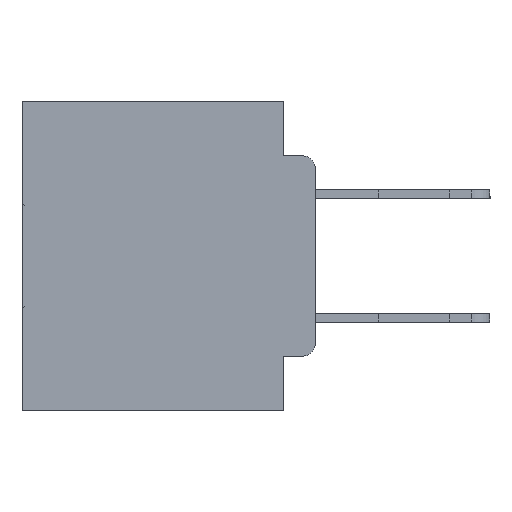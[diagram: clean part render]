
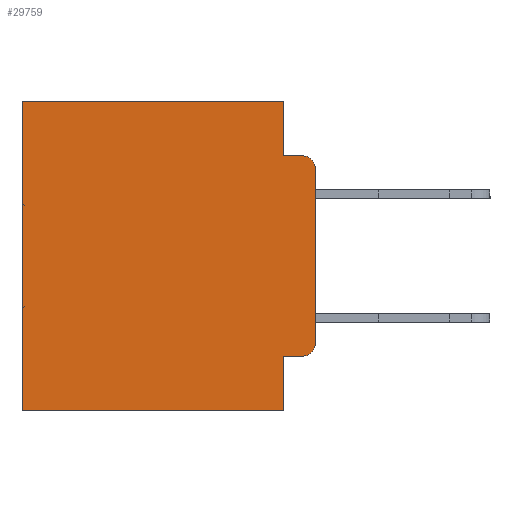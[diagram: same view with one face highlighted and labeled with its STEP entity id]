
A CAD part, left-side view. The second image highlights one B-rep face of the part: STEP entity #29759.
In plain terms, the highlighted planar face has unit normal (-1, 0, 0).
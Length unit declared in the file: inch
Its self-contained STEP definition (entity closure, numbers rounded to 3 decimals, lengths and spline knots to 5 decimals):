
#128 = EDGE_CURVE ( 'NONE', #27469, #11849, #14133, .T. ) ;
#527 = EDGE_CURVE ( 'NONE', #28524, #11849, #22527, .T. ) ;
#592 = VECTOR ( 'NONE', #29927, 39.37008 ) ;
#856 = PLANE ( 'NONE',  #10819 ) ;
#978 = LINE ( 'NONE', #7928, #26305 ) ;
#1054 = EDGE_CURVE ( 'NONE', #17844, #15784, #29932, .T. ) ;
#1127 = DIRECTION ( 'NONE',  ( 0., 0., -1. ) ) ;
#1215 = VERTEX_POINT ( 'NONE', #1244 ) ;
#1244 = CARTESIAN_POINT ( 'NONE',  ( 0.298, 0.473, -0.5 ) ) ;
#1388 = EDGE_CURVE ( 'NONE', #15784, #13657, #13635, .T. ) ;
#1436 = DIRECTION ( 'NONE',  ( 0., 0., -1. ) ) ;
#1456 = LINE ( 'NONE', #21201, #28298 ) ;
#1610 = AXIS2_PLACEMENT_3D ( 'NONE', #18810, #2027, #1436 ) ;
#1756 = CARTESIAN_POINT ( 'NONE',  ( 0.298, 0., 0. ) ) ;
#2012 = EDGE_CURVE ( 'NONE', #23651, #12272, #1456, .T. ) ;
#2027 = DIRECTION ( 'NONE',  ( -1., 0., 0. ) ) ;
#3359 = CARTESIAN_POINT ( 'NONE',  ( 0.298, 0., -0.3915 ) ) ;
#5208 = CARTESIAN_POINT ( 'NONE',  ( 0.298, 0., -0.5 ) ) ;
#5231 = DIRECTION ( 'NONE',  ( 0., 1., 0. ) ) ;
#6054 = AXIS2_PLACEMENT_3D ( 'NONE', #12619, #30339, #15205 ) ;
#7904 = DIRECTION ( 'NONE',  ( 0., 1., 0. ) ) ;
#7928 = CARTESIAN_POINT ( 'NONE',  ( 0.298, 0., 0. ) ) ;
#8842 = VERTEX_POINT ( 'NONE', #31891 ) ;
#9017 = ORIENTED_EDGE ( 'NONE', *, *, #1388, .F. ) ;
#9561 = VECTOR ( 'NONE', #24460, 39.37008 ) ;
#10523 = CARTESIAN_POINT ( 'NONE',  ( 0.298, 0.02, -0.0885 ) ) ;
#10819 = AXIS2_PLACEMENT_3D ( 'NONE', #16819, #27008, #11722 ) ;
#11003 = EDGE_CURVE ( 'NONE', #23651, #27469, #25296, .T. ) ;
#11676 = VECTOR ( 'NONE', #23609, 39.37008 ) ;
#11722 = DIRECTION ( 'NONE',  ( 0., 0., -1. ) ) ;
#11849 = VERTEX_POINT ( 'NONE', #3359 ) ;
#12272 = VERTEX_POINT ( 'NONE', #17216 ) ;
#12349 = CARTESIAN_POINT ( 'NONE',  ( 0.298, 0.051, 0. ) ) ;
#12554 = EDGE_CURVE ( 'NONE', #12272, #1215, #20875, .T. ) ;
#12619 = CARTESIAN_POINT ( 'NONE',  ( 0.298, 0.02, -0.1085 ) ) ;
#13036 = ORIENTED_EDGE ( 'NONE', *, *, #12554, .F. ) ;
#13238 = EDGE_LOOP ( 'NONE', ( #26801, #25146, #9017, #17863, #20522, #26569, #13036, #20979, #18290, #15002 ) ) ;
#13635 = LINE ( 'NONE', #22739, #26387 ) ;
#13657 = VERTEX_POINT ( 'NONE', #10523 ) ;
#14133 = CIRCLE ( 'NONE', #1610, 0.02 ) ;
#15002 = ORIENTED_EDGE ( 'NONE', *, *, #128, .T. ) ;
#15205 = DIRECTION ( 'NONE',  ( 0., 0., -1. ) ) ;
#15716 = VECTOR ( 'NONE', #32960, 39.37008 ) ;
#15784 = VERTEX_POINT ( 'NONE', #16640 ) ;
#16483 = LINE ( 'NONE', #27432, #592 ) ;
#16640 = CARTESIAN_POINT ( 'NONE',  ( 0.298, 0.051, -0.0885 ) ) ;
#16819 = CARTESIAN_POINT ( 'NONE',  ( 0.298, 0., 0. ) ) ;
#17216 = CARTESIAN_POINT ( 'NONE',  ( 0.298, 0.051, -0.5 ) ) ;
#17844 = VERTEX_POINT ( 'NONE', #12349 ) ;
#17863 = ORIENTED_EDGE ( 'NONE', *, *, #1054, .F. ) ;
#18290 = ORIENTED_EDGE ( 'NONE', *, *, #11003, .T. ) ;
#18810 = CARTESIAN_POINT ( 'NONE',  ( 0.298, 0.02, -0.3915 ) ) ;
#18944 = CARTESIAN_POINT ( 'NONE',  ( 0.298, 0., -0.1085 ) ) ;
#19044 = CIRCLE ( 'NONE', #6054, 0.02 ) ;
#20122 = VECTOR ( 'NONE', #7904, 39.37008 ) ;
#20522 = ORIENTED_EDGE ( 'NONE', *, *, #24615, .T. ) ;
#20875 = LINE ( 'NONE', #5208, #20122 ) ;
#20979 = ORIENTED_EDGE ( 'NONE', *, *, #2012, .F. ) ;
#21057 = CARTESIAN_POINT ( 'NONE',  ( 0.298, 0.051, -0.4115 ) ) ;
#21201 = CARTESIAN_POINT ( 'NONE',  ( 0.298, 0.051, 0. ) ) ;
#22527 = LINE ( 'NONE', #1756, #15716 ) ;
#22739 = CARTESIAN_POINT ( 'NONE',  ( 0.298, 0.051, -0.0885 ) ) ;
#23609 = DIRECTION ( 'NONE',  ( 0., -1., 0. ) ) ;
#23651 = VERTEX_POINT ( 'NONE', #27700 ) ;
#24317 = DIRECTION ( 'NONE',  ( 0., -1., 0. ) ) ;
#24460 = DIRECTION ( 'NONE',  ( 0., 0., -1. ) ) ;
#24615 = EDGE_CURVE ( 'NONE', #17844, #8842, #978, .T. ) ;
#25146 = ORIENTED_EDGE ( 'NONE', *, *, #27056, .T. ) ;
#25296 = LINE ( 'NONE', #21057, #11676 ) ;
#25441 = CARTESIAN_POINT ( 'NONE',  ( 0.298, 0.051, 0. ) ) ;
#26305 = VECTOR ( 'NONE', #5231, 39.37008 ) ;
#26387 = VECTOR ( 'NONE', #24317, 39.37008 ) ;
#26569 = ORIENTED_EDGE ( 'NONE', *, *, #29859, .T. ) ;
#26801 = ORIENTED_EDGE ( 'NONE', *, *, #527, .F. ) ;
#27008 = DIRECTION ( 'NONE',  ( 1., 0., 0. ) ) ;
#27056 = EDGE_CURVE ( 'NONE', #28524, #13657, #19044, .T. ) ;
#27432 = CARTESIAN_POINT ( 'NONE',  ( 0.298, 0.473, 0. ) ) ;
#27469 = VERTEX_POINT ( 'NONE', #31844 ) ;
#27700 = CARTESIAN_POINT ( 'NONE',  ( 0.298, 0.051, -0.4115 ) ) ;
#28298 = VECTOR ( 'NONE', #1127, 39.37008 ) ;
#28524 = VERTEX_POINT ( 'NONE', #18944 ) ;
#29759 = ADVANCED_FACE ( 'NONE', ( #31456 ), #856, .F. ) ;
#29859 = EDGE_CURVE ( 'NONE', #8842, #1215, #16483, .T. ) ;
#29927 = DIRECTION ( 'NONE',  ( 0., 0., -1. ) ) ;
#29932 = LINE ( 'NONE', #25441, #9561 ) ;
#30339 = DIRECTION ( 'NONE',  ( -1., 0., 0. ) ) ;
#31456 = FACE_OUTER_BOUND ( 'NONE', #13238, .T. ) ;
#31844 = CARTESIAN_POINT ( 'NONE',  ( 0.298, 0.02, -0.4115 ) ) ;
#31891 = CARTESIAN_POINT ( 'NONE',  ( 0.298, 0.473, 0. ) ) ;
#32960 = DIRECTION ( 'NONE',  ( 0., 0., -1. ) ) ;
